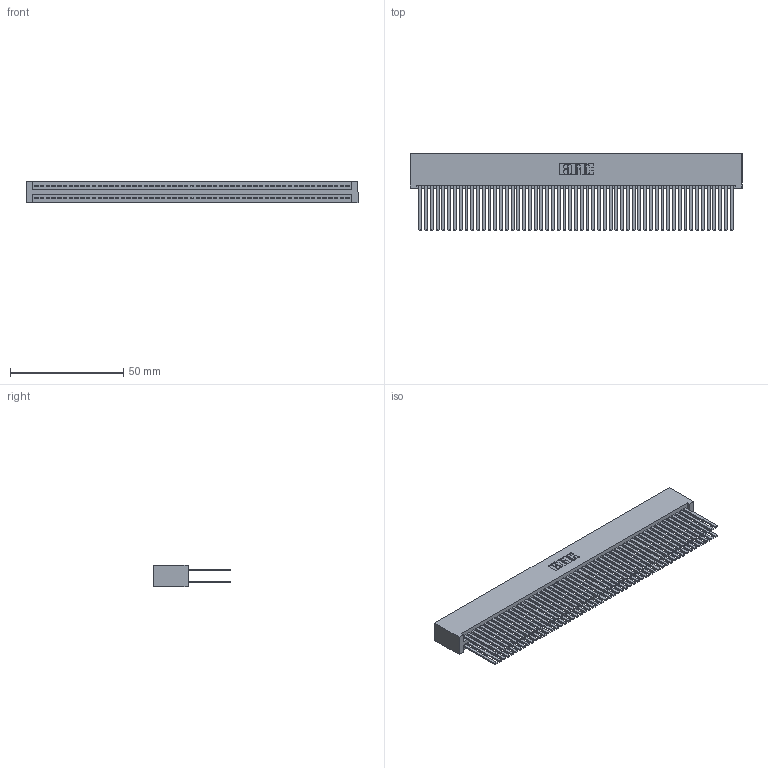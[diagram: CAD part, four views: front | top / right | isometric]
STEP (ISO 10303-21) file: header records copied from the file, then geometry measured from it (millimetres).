
FILE_DESCRIPTION (( 'STEP AP203' ), '1' );
FILE_NAME ('395-110-544-201.STEP', '2018-12-01T03:59:48', ( '' ), ( '' ), 'SwSTEP 2.0', 'SolidWorks 2016', '' );
FILE_SCHEMA (( 'CONFIG_CONTROL_DESIGN' ));
Length unit declared in the file: inch
Products named in the file (3): 345-292-001_345-293-144; 345 Part_No Mounting Lugs; 395-110-544-201
Assembly tree (111 placements, depth 2):
  395-110-544-201
    345 Part_No Mounting Lugs
    345-292-001_345-293-144  x110
Bounding box: 146.3 x 33.96 x 9.4 mm (x, y, z)
Volume: 16490.7 mm3; surface area: 29450.5 mm2
Topology: 111 solids, 111 shells, 4958 faces, 14727 edges, 9670 vertices
Faces by surface type: plane 3266, cylinder 1692
Entity records: 40943 total; most frequent: CARTESIAN_POINT 6848, ORIENTED_EDGE 6782, DIRECTION 6015, EDGE_CURVE 3391, LINE 3051, VECTOR 3051, VERTEX_POINT 2258, AXIS2_PLACEMENT_3D 1482
